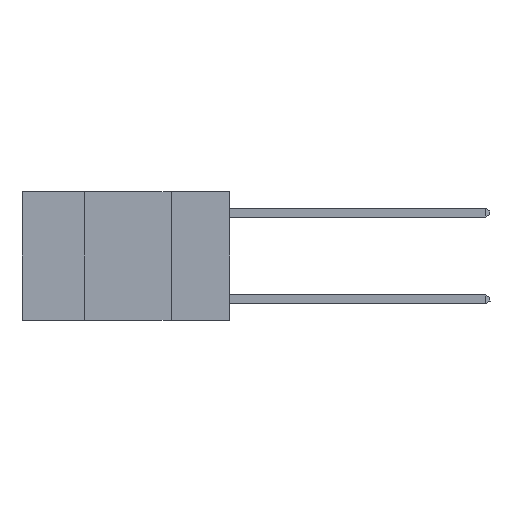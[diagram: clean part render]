
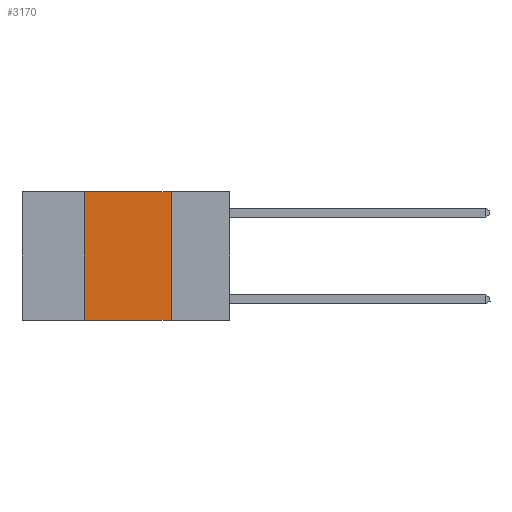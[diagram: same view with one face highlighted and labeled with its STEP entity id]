
A CAD part, left-side view. The second image highlights one B-rep face of the part: STEP entity #3170.
In plain terms, the highlighted planar face has unit normal (-1, 0, 0).
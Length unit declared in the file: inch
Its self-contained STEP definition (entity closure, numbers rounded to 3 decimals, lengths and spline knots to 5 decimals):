
#58 = EDGE_CURVE ( 'NONE', #6646, #2820, #8974, .T. ) ;
#628 = ORIENTED_EDGE ( 'NONE', *, *, #6877, .F. ) ;
#740 = EDGE_CURVE ( 'NONE', #6331, #807, #11904, .T. ) ;
#807 = VERTEX_POINT ( 'NONE', #5870 ) ;
#917 = EDGE_CURVE ( 'NONE', #6331, #6646, #8950, .T. ) ;
#960 = ORIENTED_EDGE ( 'NONE', *, *, #917, .F. ) ;
#1117 = CARTESIAN_POINT ( 'NONE',  ( 0., 0.17, 0. ) ) ;
#1139 = AXIS2_PLACEMENT_3D ( 'NONE', #9089, #3834, #11224 ) ;
#1760 = DIRECTION ( 'NONE',  ( 0., 0., -1. ) ) ;
#2370 = CARTESIAN_POINT ( 'NONE',  ( 0., 0.6, 0. ) ) ;
#2790 = PLANE ( 'NONE',  #1139 ) ;
#2820 = VERTEX_POINT ( 'NONE', #1117 ) ;
#2852 = CARTESIAN_POINT ( 'NONE',  ( 0., 0.42, -0.37 ) ) ;
#3170 = ADVANCED_FACE ( 'NONE', ( #11528 ), #2790, .F. ) ;
#3476 = ORIENTED_EDGE ( 'NONE', *, *, #58, .F. ) ;
#3790 = ORIENTED_EDGE ( 'NONE', *, *, #740, .T. ) ;
#3834 = DIRECTION ( 'NONE',  ( 1., 0., 0. ) ) ;
#4523 = CARTESIAN_POINT ( 'NONE',  ( 0., 0.42, 0. ) ) ;
#5404 = DIRECTION ( 'NONE',  ( 0., 0., 1. ) ) ;
#5870 = CARTESIAN_POINT ( 'NONE',  ( 0., 0.17, -0.37 ) ) ;
#5979 = CARTESIAN_POINT ( 'NONE',  ( 0., 0.42, 0. ) ) ;
#6331 = VERTEX_POINT ( 'NONE', #2852 ) ;
#6466 = VECTOR ( 'NONE', #5404, 39.37008 ) ;
#6646 = VERTEX_POINT ( 'NONE', #4523 ) ;
#6877 = EDGE_CURVE ( 'NONE', #2820, #807, #12513, .T. ) ;
#7137 = EDGE_LOOP ( 'NONE', ( #628, #3476, #960, #3790 ) ) ;
#7980 = DIRECTION ( 'NONE',  ( 0., -1., 0. ) ) ;
#8950 = LINE ( 'NONE', #5979, #6466 ) ;
#8974 = LINE ( 'NONE', #2370, #11123 ) ;
#9089 = CARTESIAN_POINT ( 'NONE',  ( 0., 0.6, 0. ) ) ;
#9090 = CARTESIAN_POINT ( 'NONE',  ( 0., 0.17, 0. ) ) ;
#9777 = VECTOR ( 'NONE', #1760, 39.37008 ) ;
#9904 = DIRECTION ( 'NONE',  ( 0., -1., 0. ) ) ;
#11123 = VECTOR ( 'NONE', #9904, 39.37008 ) ;
#11224 = DIRECTION ( 'NONE',  ( 0., 0., -1. ) ) ;
#11528 = FACE_OUTER_BOUND ( 'NONE', #7137, .T. ) ;
#11577 = VECTOR ( 'NONE', #7980, 39.37008 ) ;
#11904 = LINE ( 'NONE', #13290, #11577 ) ;
#12513 = LINE ( 'NONE', #9090, #9777 ) ;
#13290 = CARTESIAN_POINT ( 'NONE',  ( 0., 0.6, -0.37 ) ) ;
